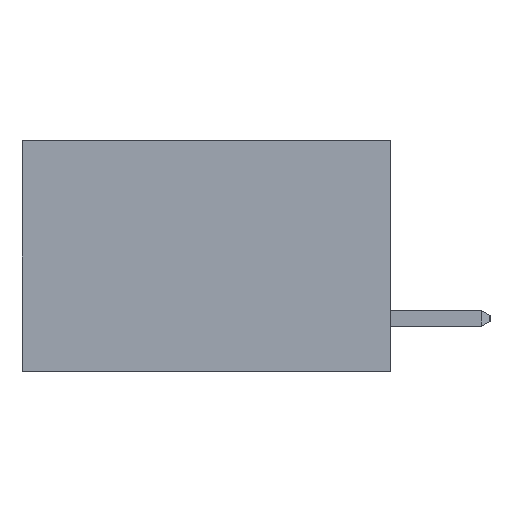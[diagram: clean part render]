
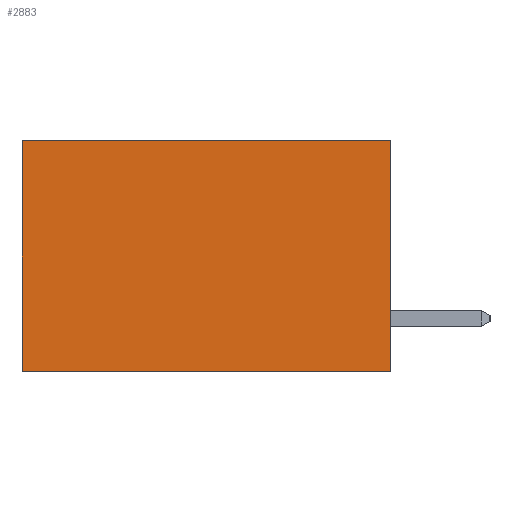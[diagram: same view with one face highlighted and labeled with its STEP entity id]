
A CAD part, left-side view. The second image highlights one B-rep face of the part: STEP entity #2883.
In plain terms, the highlighted planar face has unit normal (-1, 0, 0).
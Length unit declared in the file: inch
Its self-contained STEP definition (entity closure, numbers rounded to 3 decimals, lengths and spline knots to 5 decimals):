
#313 = LINE ( 'NONE', #5392, #3520 ) ;
#329 = CARTESIAN_POINT ( 'NONE',  ( 0.277, 0.59, 0. ) ) ;
#2182 = DIRECTION ( 'NONE',  ( 0., 1., 0. ) ) ;
#2883 = ADVANCED_FACE ( 'NONE', ( #8872 ), #14549, .F. ) ;
#3502 = CARTESIAN_POINT ( 'NONE',  ( 0.277, 0., 0. ) ) ;
#3511 = VECTOR ( 'NONE', #17477, 39.37008 ) ;
#3520 = VECTOR ( 'NONE', #2182, 39.37008 ) ;
#3694 = LINE ( 'NONE', #5276, #7851 ) ;
#4875 = ORIENTED_EDGE ( 'NONE', *, *, #10084, .T. ) ;
#5276 = CARTESIAN_POINT ( 'NONE',  ( 0.277, 0.59, -0.37 ) ) ;
#5392 = CARTESIAN_POINT ( 'NONE',  ( 0.277, 0., -0.37 ) ) ;
#5570 = CARTESIAN_POINT ( 'NONE',  ( 0.277, 0., -0.37 ) ) ;
#7758 = VERTEX_POINT ( 'NONE', #329 ) ;
#7851 = VECTOR ( 'NONE', #12984, 39.37008 ) ;
#8073 = VERTEX_POINT ( 'NONE', #3502 ) ;
#8747 = ORIENTED_EDGE ( 'NONE', *, *, #9549, .F. ) ;
#8756 = DIRECTION ( 'NONE',  ( 0., 0., -1. ) ) ;
#8872 = FACE_OUTER_BOUND ( 'NONE', #11846, .T. ) ;
#9359 = DIRECTION ( 'NONE',  ( 1., 0., 0. ) ) ;
#9549 = EDGE_CURVE ( 'NONE', #8073, #15843, #12970, .T. ) ;
#10084 = EDGE_CURVE ( 'NONE', #8073, #7758, #15333, .T. ) ;
#10105 = CARTESIAN_POINT ( 'NONE',  ( 0.277, 0.59, -0.37 ) ) ;
#10289 = ORIENTED_EDGE ( 'NONE', *, *, #18094, .T. ) ;
#10426 = ORIENTED_EDGE ( 'NONE', *, *, #15572, .F. ) ;
#10705 = VERTEX_POINT ( 'NONE', #10105 ) ;
#11468 = CARTESIAN_POINT ( 'NONE',  ( 0.277, 0., 0. ) ) ;
#11675 = CARTESIAN_POINT ( 'NONE',  ( 0.277, 0., -0.37 ) ) ;
#11846 = EDGE_LOOP ( 'NONE', ( #10289, #10426, #8747, #4875 ) ) ;
#12152 = CARTESIAN_POINT ( 'NONE',  ( 0.277, 0., -0.37 ) ) ;
#12970 = LINE ( 'NONE', #5570, #16989 ) ;
#12984 = DIRECTION ( 'NONE',  ( 0., 0., -1. ) ) ;
#13265 = DIRECTION ( 'NONE',  ( 0., 0., -1. ) ) ;
#13281 = AXIS2_PLACEMENT_3D ( 'NONE', #11675, #9359, #8756 ) ;
#14549 = PLANE ( 'NONE',  #13281 ) ;
#15333 = LINE ( 'NONE', #11468, #3511 ) ;
#15572 = EDGE_CURVE ( 'NONE', #15843, #10705, #313, .T. ) ;
#15843 = VERTEX_POINT ( 'NONE', #12152 ) ;
#16989 = VECTOR ( 'NONE', #13265, 39.37008 ) ;
#17477 = DIRECTION ( 'NONE',  ( 0., 1., 0. ) ) ;
#18094 = EDGE_CURVE ( 'NONE', #7758, #10705, #3694, .T. ) ;
